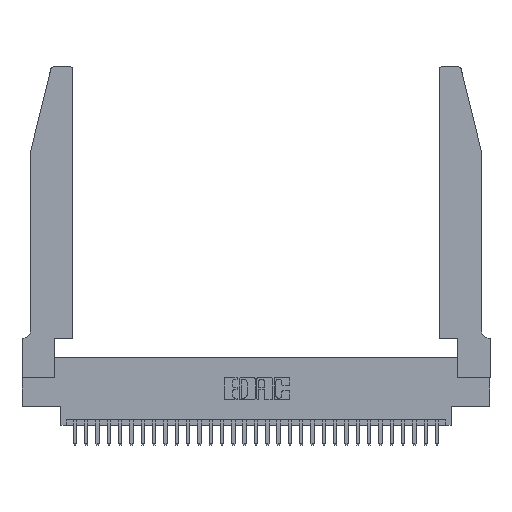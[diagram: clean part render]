
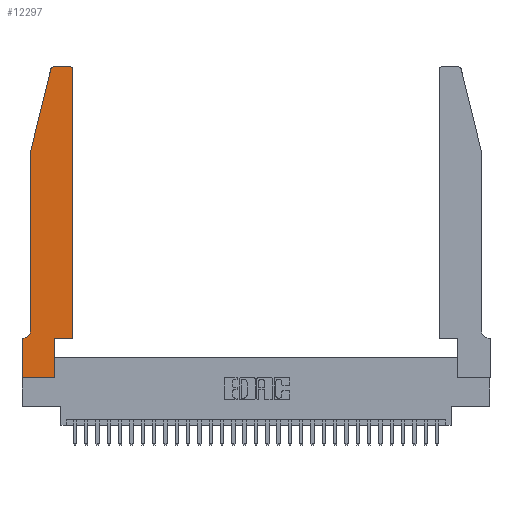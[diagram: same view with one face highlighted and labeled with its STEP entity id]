
A CAD part, top view. The second image highlights one B-rep face of the part: STEP entity #12297.
In plain terms, the highlighted planar face has unit normal (0, 0, 1).
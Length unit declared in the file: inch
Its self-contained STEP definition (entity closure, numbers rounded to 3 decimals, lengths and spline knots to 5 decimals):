
#267 = DIRECTION ( 'NONE',  ( 0., 0., -1. ) ) ;
#646 = CARTESIAN_POINT ( 'NONE',  ( 0.4205, 2.75, 0.37 ) ) ;
#685 = PLANE ( 'NONE',  #14957 ) ;
#1559 = VECTOR ( 'NONE', #2999, 39.37008 ) ;
#1905 = DIRECTION ( 'NONE',  ( 0., -1., 0. ) ) ;
#2017 = CARTESIAN_POINT ( 'NONE',  ( 0.0755, 0.35, 0.37 ) ) ;
#2085 = VECTOR ( 'NONE', #4540, 39.37008 ) ;
#2481 = CARTESIAN_POINT ( 'NONE',  ( 0.2865, 0.35, 0.37 ) ) ;
#2777 = EDGE_CURVE ( 'NONE', #9546, #26000, #29648, .T. ) ;
#2999 = DIRECTION ( 'NONE',  ( -0.239, -0.971, 0. ) ) ;
#3171 = DIRECTION ( 'NONE',  ( 0., 0., 1. ) ) ;
#3267 = EDGE_LOOP ( 'NONE', ( #22379, #17382, #25509, #13938, #22017, #28613, #17012, #12002, #13554, #15100, #10055, #11626 ) ) ;
#4214 = CARTESIAN_POINT ( 'NONE',  ( 0.4505, 0.35, 0.37 ) ) ;
#4506 = VERTEX_POINT ( 'NONE', #5855 ) ;
#4540 = DIRECTION ( 'NONE',  ( -1., 0., 0. ) ) ;
#4581 = EDGE_CURVE ( 'NONE', #29920, #8930, #30295, .T. ) ;
#4675 = EDGE_CURVE ( 'NONE', #10609, #25323, #14078, .T. ) ;
#4999 = DIRECTION ( 'NONE',  ( 0., 1., 0. ) ) ;
#5498 = VECTOR ( 'NONE', #18430, 39.37008 ) ;
#5855 = CARTESIAN_POINT ( 'NONE',  ( 0.2865, 0.35, 0.37 ) ) ;
#7041 = CARTESIAN_POINT ( 'NONE',  ( 0.0755, 2., 0.37 ) ) ;
#7248 = EDGE_CURVE ( 'NONE', #26000, #10609, #20804, .T. ) ;
#8532 = EDGE_CURVE ( 'NONE', #25323, #26595, #29659, .T. ) ;
#8832 = EDGE_CURVE ( 'NONE', #28675, #29920, #21883, .T. ) ;
#8930 = VERTEX_POINT ( 'NONE', #19824 ) ;
#8993 = LINE ( 'NONE', #15434, #1559 ) ;
#9224 = CARTESIAN_POINT ( 'NONE',  ( 0.284, 2.75, 0.37 ) ) ;
#9546 = VERTEX_POINT ( 'NONE', #4214 ) ;
#9643 = EDGE_CURVE ( 'NONE', #11109, #16545, #13030, .T. ) ;
#9940 = LINE ( 'NONE', #10477, #28117 ) ;
#10055 = ORIENTED_EDGE ( 'NONE', *, *, #2777, .T. ) ;
#10477 = CARTESIAN_POINT ( 'NONE',  ( 0., 0., 0.37 ) ) ;
#10609 = VERTEX_POINT ( 'NONE', #646 ) ;
#10623 = CARTESIAN_POINT ( 'NONE',  ( 0.4205, 2.72, 0.37 ) ) ;
#10994 = DIRECTION ( 'NONE',  ( 0., 0., 1. ) ) ;
#11047 = CARTESIAN_POINT ( 'NONE',  ( 0.2865, 0., 0.37 ) ) ;
#11109 = VERTEX_POINT ( 'NONE', #30236 ) ;
#11225 = FACE_OUTER_BOUND ( 'NONE', #3267, .T. ) ;
#11626 = ORIENTED_EDGE ( 'NONE', *, *, #7248, .T. ) ;
#12002 = ORIENTED_EDGE ( 'NONE', *, *, #32117, .T. ) ;
#12297 = ADVANCED_FACE ( 'NONE', ( #11225 ), #685, .T. ) ;
#13030 = LINE ( 'NONE', #7041, #25374 ) ;
#13132 = DIRECTION ( 'NONE',  ( 1., 0., 0. ) ) ;
#13337 = CIRCLE ( 'NONE', #13690, 0.07 ) ;
#13554 = ORIENTED_EDGE ( 'NONE', *, *, #22601, .T. ) ;
#13603 = CARTESIAN_POINT ( 'NONE',  ( 0., 0., 0.37 ) ) ;
#13690 = AXIS2_PLACEMENT_3D ( 'NONE', #15195, #267, #17668 ) ;
#13861 = CARTESIAN_POINT ( 'NONE',  ( 0.0755, 0.42, 0.37 ) ) ;
#13938 = ORIENTED_EDGE ( 'NONE', *, *, #9643, .T. ) ;
#14078 = LINE ( 'NONE', #18867, #26430 ) ;
#14160 = CARTESIAN_POINT ( 'NONE',  ( 0.25487, 2.72718, 0.37 ) ) ;
#14957 = AXIS2_PLACEMENT_3D ( 'NONE', #30398, #3171, #20540 ) ;
#15100 = ORIENTED_EDGE ( 'NONE', *, *, #21119, .T. ) ;
#15195 = CARTESIAN_POINT ( 'NONE',  ( 0.0055, 0.42, 0.37 ) ) ;
#15434 = CARTESIAN_POINT ( 'NONE',  ( 0.0755, 2., 0.37 ) ) ;
#15502 = DIRECTION ( 'NONE',  ( 0., 1., 0. ) ) ;
#16545 = VERTEX_POINT ( 'NONE', #13861 ) ;
#16726 = DIRECTION ( 'NONE',  ( 1., 0., 0. ) ) ;
#17012 = ORIENTED_EDGE ( 'NONE', *, *, #4581, .T. ) ;
#17382 = ORIENTED_EDGE ( 'NONE', *, *, #8532, .T. ) ;
#17668 = DIRECTION ( 'NONE',  ( -1., 0., 0. ) ) ;
#18430 = DIRECTION ( 'NONE',  ( 0., -1., 0. ) ) ;
#18867 = CARTESIAN_POINT ( 'NONE',  ( 0.2605, 2.75, 0.37 ) ) ;
#19824 = CARTESIAN_POINT ( 'NONE',  ( 0., 0., 0.37 ) ) ;
#20540 = DIRECTION ( 'NONE',  ( 1., 0., 0. ) ) ;
#20804 = CIRCLE ( 'NONE', #21229, 0.03 ) ;
#21119 = EDGE_CURVE ( 'NONE', #4506, #9546, #27649, .T. ) ;
#21229 = AXIS2_PLACEMENT_3D ( 'NONE', #10623, #27913, #13132 ) ;
#21371 = EDGE_CURVE ( 'NONE', #16545, #28675, #13337, .T. ) ;
#21660 = CARTESIAN_POINT ( 'NONE',  ( 0.4505, 0.35, 0.37 ) ) ;
#21883 = LINE ( 'NONE', #2017, #2085 ) ;
#22017 = ORIENTED_EDGE ( 'NONE', *, *, #21371, .T. ) ;
#22094 = AXIS2_PLACEMENT_3D ( 'NONE', #25790, #10994, #28272 ) ;
#22379 = ORIENTED_EDGE ( 'NONE', *, *, #4675, .T. ) ;
#22601 = EDGE_CURVE ( 'NONE', #29909, #4506, #25657, .T. ) ;
#25323 = VERTEX_POINT ( 'NONE', #9224 ) ;
#25374 = VECTOR ( 'NONE', #1905, 39.37008 ) ;
#25509 = ORIENTED_EDGE ( 'NONE', *, *, #28299, .T. ) ;
#25657 = LINE ( 'NONE', #2481, #30688 ) ;
#25790 = CARTESIAN_POINT ( 'NONE',  ( 0.284, 2.72, 0.37 ) ) ;
#25840 = CARTESIAN_POINT ( 'NONE',  ( 0., 0.35, 0.37 ) ) ;
#26000 = VERTEX_POINT ( 'NONE', #26713 ) ;
#26338 = DIRECTION ( 'NONE',  ( -1., 0., 0. ) ) ;
#26430 = VECTOR ( 'NONE', #26338, 39.37008 ) ;
#26595 = VERTEX_POINT ( 'NONE', #14160 ) ;
#26713 = CARTESIAN_POINT ( 'NONE',  ( 0.4505, 2.72, 0.37 ) ) ;
#26887 = VECTOR ( 'NONE', #16726, 39.37008 ) ;
#27649 = LINE ( 'NONE', #21660, #26887 ) ;
#27809 = CARTESIAN_POINT ( 'NONE',  ( 0.4505, 0.35, 0.37 ) ) ;
#27913 = DIRECTION ( 'NONE',  ( 0., 0., 1. ) ) ;
#28117 = VECTOR ( 'NONE', #30254, 39.37008 ) ;
#28272 = DIRECTION ( 'NONE',  ( 1., 0., 0. ) ) ;
#28299 = EDGE_CURVE ( 'NONE', #26595, #11109, #8993, .T. ) ;
#28613 = ORIENTED_EDGE ( 'NONE', *, *, #8832, .T. ) ;
#28675 = VERTEX_POINT ( 'NONE', #31635 ) ;
#28865 = VECTOR ( 'NONE', #15502, 39.37008 ) ;
#29648 = LINE ( 'NONE', #27809, #28865 ) ;
#29659 = CIRCLE ( 'NONE', #22094, 0.03 ) ;
#29909 = VERTEX_POINT ( 'NONE', #11047 ) ;
#29920 = VERTEX_POINT ( 'NONE', #25840 ) ;
#30236 = CARTESIAN_POINT ( 'NONE',  ( 0.0755, 2., 0.37 ) ) ;
#30254 = DIRECTION ( 'NONE',  ( 1., 0., 0. ) ) ;
#30295 = LINE ( 'NONE', #13603, #5498 ) ;
#30398 = CARTESIAN_POINT ( 'NONE',  ( 0., 0.35, 0.37 ) ) ;
#30688 = VECTOR ( 'NONE', #4999, 39.37008 ) ;
#31635 = CARTESIAN_POINT ( 'NONE',  ( 0.0055, 0.35, 0.37 ) ) ;
#32117 = EDGE_CURVE ( 'NONE', #8930, #29909, #9940, .T. ) ;
